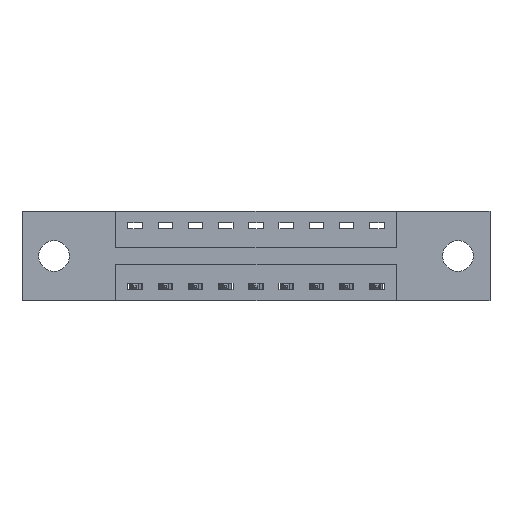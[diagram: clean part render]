
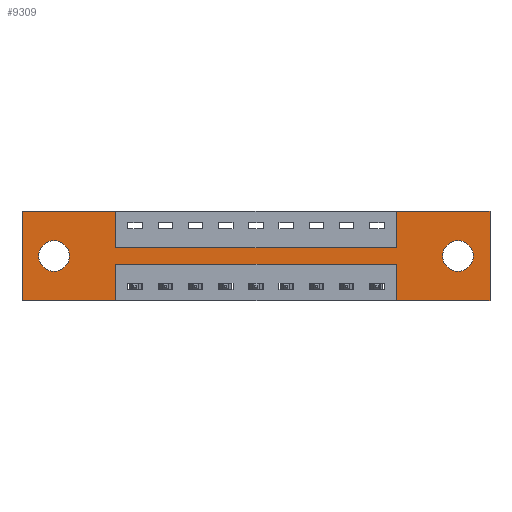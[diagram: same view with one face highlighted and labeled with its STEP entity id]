
A CAD part, front view. The second image highlights one B-rep face of the part: STEP entity #9309.
In plain terms, the highlighted planar face has unit normal (0, -1, 0).
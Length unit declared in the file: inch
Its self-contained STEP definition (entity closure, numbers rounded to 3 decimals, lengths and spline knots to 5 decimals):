
#3 = VECTOR ( 'NONE', #6579, 39.37008 ) ;
#25 = EDGE_CURVE ( 'NONE', #9441, #7542, #3726, .T. ) ;
#92 = DIRECTION ( 'NONE',  ( 0., 0., -1. ) ) ;
#107 = EDGE_CURVE ( 'NONE', #9040, #4875, #7364, .T. ) ;
#151 = ORIENTED_EDGE ( 'NONE', *, *, #8499, .T. ) ;
#166 = VECTOR ( 'NONE', #4345, 39.37008 ) ;
#185 = CARTESIAN_POINT ( 'NONE',  ( 0.3875, 0., 0. ) ) ;
#229 = ORIENTED_EDGE ( 'NONE', *, *, #1185, .F. ) ;
#360 = DIRECTION ( 'NONE',  ( 0., 0., 1. ) ) ;
#396 = CARTESIAN_POINT ( 'NONE',  ( 0., 0., 0. ) ) ;
#427 = VERTEX_POINT ( 'NONE', #396 ) ;
#483 = EDGE_CURVE ( 'NONE', #868, #8280, #5546, .T. ) ;
#524 = ORIENTED_EDGE ( 'NONE', *, *, #2025, .F. ) ;
#752 = VERTEX_POINT ( 'NONE', #9225 ) ;
#761 = LINE ( 'NONE', #6441, #4639 ) ;
#814 = ORIENTED_EDGE ( 'NONE', *, *, #4930, .F. ) ;
#868 = VERTEX_POINT ( 'NONE', #185 ) ;
#932 = VECTOR ( 'NONE', #9498, 39.37008 ) ;
#1008 = LINE ( 'NONE', #5099, #1254 ) ;
#1027 = EDGE_LOOP ( 'NONE', ( #7192, #6890 ) ) ;
#1029 = FACE_BOUND ( 'NONE', #1027, .T. ) ;
#1046 = CARTESIAN_POINT ( 'NONE',  ( 1.5475, 0., -0.37 ) ) ;
#1185 = EDGE_CURVE ( 'NONE', #5844, #9040, #7589, .T. ) ;
#1195 = AXIS2_PLACEMENT_3D ( 'NONE', #2463, #7879, #3245 ) ;
#1254 = VECTOR ( 'NONE', #9713, 39.37008 ) ;
#1385 = VERTEX_POINT ( 'NONE', #8548 ) ;
#1455 = CARTESIAN_POINT ( 'NONE',  ( 0., 0., -0.37 ) ) ;
#1504 = LINE ( 'NONE', #5333, #3322 ) ;
#1597 = VERTEX_POINT ( 'NONE', #6510 ) ;
#1612 = DIRECTION ( 'NONE',  ( 0., 1., 0. ) ) ;
#1737 = ORIENTED_EDGE ( 'NONE', *, *, #107, .F. ) ;
#2025 = EDGE_CURVE ( 'NONE', #427, #868, #7337, .T. ) ;
#2146 = VERTEX_POINT ( 'NONE', #3534 ) ;
#2243 = DIRECTION ( 'NONE',  ( 1., 0., 0. ) ) ;
#2279 = ORIENTED_EDGE ( 'NONE', *, *, #8272, .F. ) ;
#2331 = CARTESIAN_POINT ( 'NONE',  ( 1.935, 0., -0.37 ) ) ;
#2332 = DIRECTION ( 'NONE',  ( 0., 0., 1. ) ) ;
#2463 = CARTESIAN_POINT ( 'NONE',  ( 1.8025, 0., -0.185 ) ) ;
#2619 = DIRECTION ( 'NONE',  ( 1., 0., 0. ) ) ;
#2667 = AXIS2_PLACEMENT_3D ( 'NONE', #9209, #4569, #9995 ) ;
#2722 = CARTESIAN_POINT ( 'NONE',  ( 0.3875, 0., -0.15 ) ) ;
#2751 = CARTESIAN_POINT ( 'NONE',  ( 0., 0., -0.37 ) ) ;
#2769 = EDGE_CURVE ( 'NONE', #1597, #1385, #4099, .T. ) ;
#2804 = VERTEX_POINT ( 'NONE', #5821 ) ;
#2985 = CARTESIAN_POINT ( 'NONE',  ( 0.1325, 0., -0.185 ) ) ;
#3081 = FACE_BOUND ( 'NONE', #9614, .T. ) ;
#3107 = ORIENTED_EDGE ( 'NONE', *, *, #7821, .F. ) ;
#3177 = CIRCLE ( 'NONE', #1195, 0.064 ) ;
#3245 = DIRECTION ( 'NONE',  ( 0., 0., -1. ) ) ;
#3277 = CARTESIAN_POINT ( 'NONE',  ( 0.1325, 0., -0.249 ) ) ;
#3322 = VECTOR ( 'NONE', #9167, 39.37008 ) ;
#3385 = CARTESIAN_POINT ( 'NONE',  ( 1.5475, 0., -0.22 ) ) ;
#3395 = CARTESIAN_POINT ( 'NONE',  ( 0., 0., 0. ) ) ;
#3472 = CARTESIAN_POINT ( 'NONE',  ( 0., 0., 0. ) ) ;
#3534 = CARTESIAN_POINT ( 'NONE',  ( 0.1325, 0., -0.121 ) ) ;
#3655 = CARTESIAN_POINT ( 'NONE',  ( 0.3875, 0., -0.37 ) ) ;
#3726 = LINE ( 'NONE', #5093, #7596 ) ;
#3767 = DIRECTION ( 'NONE',  ( 0., 0., 1. ) ) ;
#4099 = LINE ( 'NONE', #8874, #5923 ) ;
#4141 = CIRCLE ( 'NONE', #7160, 0.064 ) ;
#4345 = DIRECTION ( 'NONE',  ( 0., 0., -1. ) ) ;
#4374 = LINE ( 'NONE', #3472, #3 ) ;
#4399 = ORIENTED_EDGE ( 'NONE', *, *, #7175, .T. ) ;
#4410 = DIRECTION ( 'NONE',  ( 0., 0., -1. ) ) ;
#4503 = EDGE_CURVE ( 'NONE', #6995, #752, #7937, .T. ) ;
#4555 = CARTESIAN_POINT ( 'NONE',  ( 0.3875, 0., -0.15 ) ) ;
#4569 = DIRECTION ( 'NONE',  ( 0., 1., 0. ) ) ;
#4626 = LINE ( 'NONE', #4555, #6447 ) ;
#4639 = VECTOR ( 'NONE', #7233, 39.37008 ) ;
#4737 = DIRECTION ( 'NONE',  ( 0., -1., 0. ) ) ;
#4843 = CARTESIAN_POINT ( 'NONE',  ( 0.3875, 0., -0.22 ) ) ;
#4875 = VERTEX_POINT ( 'NONE', #2751 ) ;
#4930 = EDGE_CURVE ( 'NONE', #2804, #5223, #5874, .T. ) ;
#5093 = CARTESIAN_POINT ( 'NONE',  ( 1.5475, 0., -0.37 ) ) ;
#5099 = CARTESIAN_POINT ( 'NONE',  ( 0., 0., -0.37 ) ) ;
#5124 = CARTESIAN_POINT ( 'NONE',  ( 0.3875, 0., 0. ) ) ;
#5223 = VERTEX_POINT ( 'NONE', #2331 ) ;
#5292 = VECTOR ( 'NONE', #2619, 39.37008 ) ;
#5308 = VECTOR ( 'NONE', #4410, 39.37008 ) ;
#5333 = CARTESIAN_POINT ( 'NONE',  ( 0., 0., 0. ) ) ;
#5383 = VERTEX_POINT ( 'NONE', #3277 ) ;
#5443 = ORIENTED_EDGE ( 'NONE', *, *, #7377, .F. ) ;
#5536 = EDGE_CURVE ( 'NONE', #5223, #9441, #1008, .T. ) ;
#5546 = LINE ( 'NONE', #5124, #7586 ) ;
#5656 = ORIENTED_EDGE ( 'NONE', *, *, #25, .F. ) ;
#5675 = ORIENTED_EDGE ( 'NONE', *, *, #483, .F. ) ;
#5789 = EDGE_CURVE ( 'NONE', #752, #6995, #3177, .T. ) ;
#5821 = CARTESIAN_POINT ( 'NONE',  ( 1.935, 0., 0. ) ) ;
#5844 = VERTEX_POINT ( 'NONE', #4843 ) ;
#5874 = LINE ( 'NONE', #8986, #166 ) ;
#5923 = VECTOR ( 'NONE', #360, 39.37008 ) ;
#6148 = EDGE_LOOP ( 'NONE', ( #229, #5443, #5656, #8003, #814, #9177, #7429, #3107, #5675, #524, #2279, #1737 ) ) ;
#6252 = CARTESIAN_POINT ( 'NONE',  ( 0.1325, 0., -0.185 ) ) ;
#6327 = AXIS2_PLACEMENT_3D ( 'NONE', #8605, #4737, #92 ) ;
#6441 = CARTESIAN_POINT ( 'NONE',  ( 0.3875, 0., -0.22 ) ) ;
#6447 = VECTOR ( 'NONE', #2243, 39.37008 ) ;
#6510 = CARTESIAN_POINT ( 'NONE',  ( 1.5475, 0., -0.15 ) ) ;
#6579 = DIRECTION ( 'NONE',  ( 0., 0., 1. ) ) ;
#6890 = ORIENTED_EDGE ( 'NONE', *, *, #4503, .T. ) ;
#6903 = AXIS2_PLACEMENT_3D ( 'NONE', #2985, #8398, #3767 ) ;
#6995 = VERTEX_POINT ( 'NONE', #9882 ) ;
#7021 = DIRECTION ( 'NONE',  ( 0., 0., 1. ) ) ;
#7160 = AXIS2_PLACEMENT_3D ( 'NONE', #6252, #1612, #7021 ) ;
#7175 = EDGE_CURVE ( 'NONE', #5383, #2146, #4141, .T. ) ;
#7192 = ORIENTED_EDGE ( 'NONE', *, *, #5789, .T. ) ;
#7212 = FACE_OUTER_BOUND ( 'NONE', #6148, .T. ) ;
#7233 = DIRECTION ( 'NONE',  ( -1., 0., 0. ) ) ;
#7337 = LINE ( 'NONE', #3395, #5292 ) ;
#7364 = LINE ( 'NONE', #1455, #932 ) ;
#7377 = EDGE_CURVE ( 'NONE', #7542, #5844, #761, .T. ) ;
#7429 = ORIENTED_EDGE ( 'NONE', *, *, #2769, .F. ) ;
#7542 = VERTEX_POINT ( 'NONE', #3385 ) ;
#7586 = VECTOR ( 'NONE', #9755, 39.37008 ) ;
#7589 = LINE ( 'NONE', #8271, #5308 ) ;
#7596 = VECTOR ( 'NONE', #2332, 39.37008 ) ;
#7819 = PLANE ( 'NONE',  #6327 ) ;
#7821 = EDGE_CURVE ( 'NONE', #8280, #1597, #4626, .T. ) ;
#7879 = DIRECTION ( 'NONE',  ( 0., 1., 0. ) ) ;
#7886 = CIRCLE ( 'NONE', #6903, 0.064 ) ;
#7937 = CIRCLE ( 'NONE', #2667, 0.064 ) ;
#8003 = ORIENTED_EDGE ( 'NONE', *, *, #5536, .F. ) ;
#8271 = CARTESIAN_POINT ( 'NONE',  ( 0.3875, 0., -0.37 ) ) ;
#8272 = EDGE_CURVE ( 'NONE', #4875, #427, #4374, .T. ) ;
#8280 = VERTEX_POINT ( 'NONE', #2722 ) ;
#8398 = DIRECTION ( 'NONE',  ( 0., 1., 0. ) ) ;
#8499 = EDGE_CURVE ( 'NONE', #2146, #5383, #7886, .T. ) ;
#8548 = CARTESIAN_POINT ( 'NONE',  ( 1.5475, 0., 0. ) ) ;
#8605 = CARTESIAN_POINT ( 'NONE',  ( 0., 0., -0.37 ) ) ;
#8874 = CARTESIAN_POINT ( 'NONE',  ( 1.5475, 0., 0. ) ) ;
#8986 = CARTESIAN_POINT ( 'NONE',  ( 1.935, 0., 0. ) ) ;
#9040 = VERTEX_POINT ( 'NONE', #3655 ) ;
#9167 = DIRECTION ( 'NONE',  ( 1., 0., 0. ) ) ;
#9177 = ORIENTED_EDGE ( 'NONE', *, *, #9703, .F. ) ;
#9209 = CARTESIAN_POINT ( 'NONE',  ( 1.8025, 0., -0.185 ) ) ;
#9225 = CARTESIAN_POINT ( 'NONE',  ( 1.8025, 0., -0.121 ) ) ;
#9309 = ADVANCED_FACE ( 'NONE', ( #1029, #3081, #7212 ), #7819, .T. ) ;
#9441 = VERTEX_POINT ( 'NONE', #1046 ) ;
#9498 = DIRECTION ( 'NONE',  ( -1., 0., 0. ) ) ;
#9614 = EDGE_LOOP ( 'NONE', ( #151, #4399 ) ) ;
#9703 = EDGE_CURVE ( 'NONE', #1385, #2804, #1504, .T. ) ;
#9713 = DIRECTION ( 'NONE',  ( -1., 0., 0. ) ) ;
#9755 = DIRECTION ( 'NONE',  ( 0., 0., -1. ) ) ;
#9882 = CARTESIAN_POINT ( 'NONE',  ( 1.8025, 0., -0.249 ) ) ;
#9995 = DIRECTION ( 'NONE',  ( 0., 0., -1. ) ) ;
